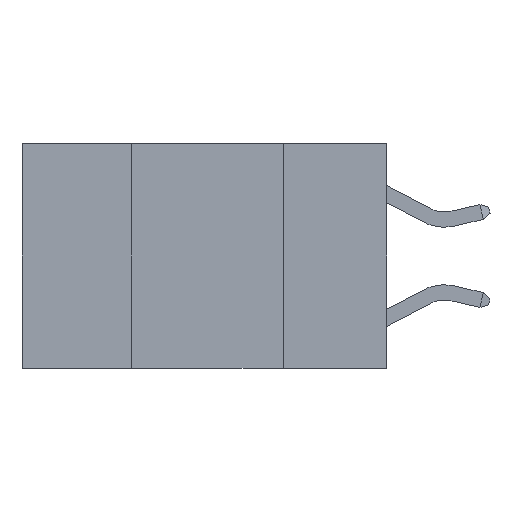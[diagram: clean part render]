
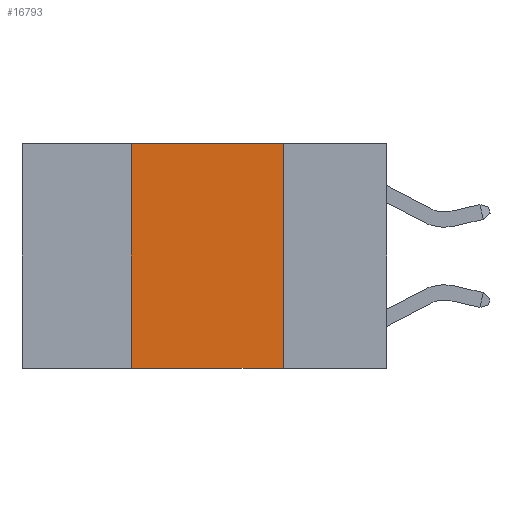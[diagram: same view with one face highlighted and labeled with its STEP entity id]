
A CAD part, left-side view. The second image highlights one B-rep face of the part: STEP entity #16793.
In plain terms, the highlighted planar face has unit normal (-1, 0, 0).
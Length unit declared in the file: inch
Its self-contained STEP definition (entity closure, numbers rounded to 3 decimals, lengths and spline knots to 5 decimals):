
#845 = ORIENTED_EDGE ( 'NONE', *, *, #6411, .F. ) ;
#870 = LINE ( 'NONE', #16825, #7694 ) ;
#1023 = AXIS2_PLACEMENT_3D ( 'NONE', #8415, #3240, #3085 ) ;
#1943 = EDGE_LOOP ( 'NONE', ( #14003, #13120, #845, #8646 ) ) ;
#2188 = CARTESIAN_POINT ( 'NONE',  ( 0., 0.42, -0.37 ) ) ;
#2386 = VECTOR ( 'NONE', #6969, 39.37008 ) ;
#2458 = LINE ( 'NONE', #7807, #8179 ) ;
#2566 = CARTESIAN_POINT ( 'NONE',  ( 0., 0.17, 0. ) ) ;
#3085 = DIRECTION ( 'NONE',  ( 0., 0., -1. ) ) ;
#3106 = VERTEX_POINT ( 'NONE', #12644 ) ;
#3132 = VERTEX_POINT ( 'NONE', #2188 ) ;
#3240 = DIRECTION ( 'NONE',  ( 1., 0., 0. ) ) ;
#3555 = DIRECTION ( 'NONE',  ( 0., -1., 0. ) ) ;
#6260 = EDGE_CURVE ( 'NONE', #3132, #3106, #17213, .T. ) ;
#6411 = EDGE_CURVE ( 'NONE', #3132, #15671, #2458, .T. ) ;
#6969 = DIRECTION ( 'NONE',  ( 0., 0., -1. ) ) ;
#6989 = VERTEX_POINT ( 'NONE', #2566 ) ;
#7694 = VECTOR ( 'NONE', #3555, 39.37008 ) ;
#7807 = CARTESIAN_POINT ( 'NONE',  ( 0., 0.42, 0. ) ) ;
#7916 = DIRECTION ( 'NONE',  ( 0., -1., 0. ) ) ;
#8179 = VECTOR ( 'NONE', #13056, 39.37008 ) ;
#8369 = LINE ( 'NONE', #12398, #2386 ) ;
#8415 = CARTESIAN_POINT ( 'NONE',  ( 0., 0.6, 0. ) ) ;
#8646 = ORIENTED_EDGE ( 'NONE', *, *, #6260, .T. ) ;
#8716 = VECTOR ( 'NONE', #7916, 39.37008 ) ;
#8917 = EDGE_CURVE ( 'NONE', #6989, #3106, #8369, .T. ) ;
#9626 = FACE_OUTER_BOUND ( 'NONE', #1943, .T. ) ;
#12398 = CARTESIAN_POINT ( 'NONE',  ( 0., 0.17, 0. ) ) ;
#12644 = CARTESIAN_POINT ( 'NONE',  ( 0., 0.17, -0.37 ) ) ;
#13056 = DIRECTION ( 'NONE',  ( 0., 0., 1. ) ) ;
#13120 = ORIENTED_EDGE ( 'NONE', *, *, #13661, .F. ) ;
#13661 = EDGE_CURVE ( 'NONE', #15671, #6989, #870, .T. ) ;
#14003 = ORIENTED_EDGE ( 'NONE', *, *, #8917, .F. ) ;
#14622 = CARTESIAN_POINT ( 'NONE',  ( 0., 0.6, -0.37 ) ) ;
#15671 = VERTEX_POINT ( 'NONE', #16336 ) ;
#16249 = PLANE ( 'NONE',  #1023 ) ;
#16336 = CARTESIAN_POINT ( 'NONE',  ( 0., 0.42, 0. ) ) ;
#16793 = ADVANCED_FACE ( 'NONE', ( #9626 ), #16249, .F. ) ;
#16825 = CARTESIAN_POINT ( 'NONE',  ( 0., 0.6, 0. ) ) ;
#17213 = LINE ( 'NONE', #14622, #8716 ) ;
